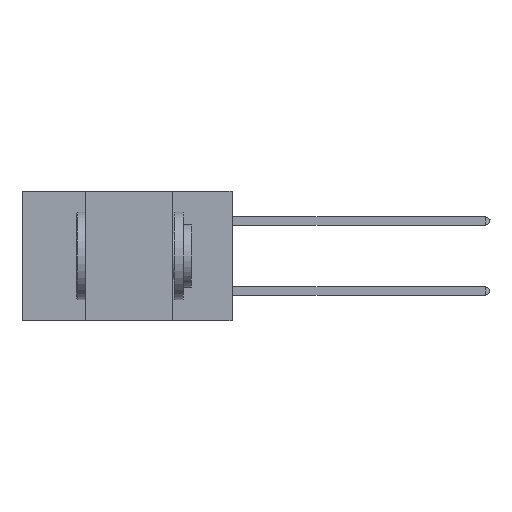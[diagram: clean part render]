
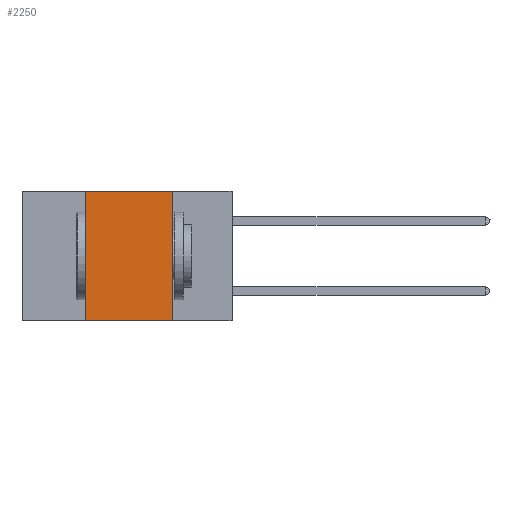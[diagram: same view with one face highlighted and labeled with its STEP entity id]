
A CAD part, left-side view. The second image highlights one B-rep face of the part: STEP entity #2250.
In plain terms, the highlighted planar face has unit normal (-1, 0, 0).
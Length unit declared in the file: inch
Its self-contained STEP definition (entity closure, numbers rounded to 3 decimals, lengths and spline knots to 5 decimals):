
#39 = CARTESIAN_POINT ( 'NONE',  ( 0., 0.17, -0.37 ) ) ;
#564 = ORIENTED_EDGE ( 'NONE', *, *, #9642, .F. ) ;
#655 = VECTOR ( 'NONE', #10500, 39.37008 ) ;
#731 = VERTEX_POINT ( 'NONE', #39 ) ;
#1164 = ORIENTED_EDGE ( 'NONE', *, *, #5326, .F. ) ;
#1680 = ORIENTED_EDGE ( 'NONE', *, *, #9008, .T. ) ;
#2250 = ADVANCED_FACE ( 'NONE', ( #8075 ), #3520, .F. ) ;
#2349 = EDGE_CURVE ( 'NONE', #7176, #6942, #9381, .T. ) ;
#2686 = DIRECTION ( 'NONE',  ( 0., 0., -1. ) ) ;
#2958 = VECTOR ( 'NONE', #10139, 39.37008 ) ;
#3029 = DIRECTION ( 'NONE',  ( 0., 0., 1. ) ) ;
#3080 = VECTOR ( 'NONE', #2686, 39.37008 ) ;
#3149 = EDGE_LOOP ( 'NONE', ( #564, #1164, #5261, #1680 ) ) ;
#3520 = PLANE ( 'NONE',  #9541 ) ;
#4089 = CARTESIAN_POINT ( 'NONE',  ( 0., 0.42, 0. ) ) ;
#4205 = CARTESIAN_POINT ( 'NONE',  ( 0., 0.42, 0. ) ) ;
#5202 = CARTESIAN_POINT ( 'NONE',  ( 0., 0.6, 0. ) ) ;
#5261 = ORIENTED_EDGE ( 'NONE', *, *, #2349, .F. ) ;
#5326 = EDGE_CURVE ( 'NONE', #6942, #9904, #7700, .T. ) ;
#5438 = LINE ( 'NONE', #7901, #3080 ) ;
#6510 = DIRECTION ( 'NONE',  ( 0., 0., -1. ) ) ;
#6512 = DIRECTION ( 'NONE',  ( 1., 0., 0. ) ) ;
#6942 = VERTEX_POINT ( 'NONE', #4205 ) ;
#7176 = VERTEX_POINT ( 'NONE', #9495 ) ;
#7332 = VECTOR ( 'NONE', #3029, 39.37008 ) ;
#7700 = LINE ( 'NONE', #9699, #655 ) ;
#7901 = CARTESIAN_POINT ( 'NONE',  ( 0., 0.17, 0. ) ) ;
#8075 = FACE_OUTER_BOUND ( 'NONE', #3149, .T. ) ;
#8216 = CARTESIAN_POINT ( 'NONE',  ( 0., 0.17, 0. ) ) ;
#9008 = EDGE_CURVE ( 'NONE', #7176, #731, #9663, .T. ) ;
#9333 = CARTESIAN_POINT ( 'NONE',  ( 0., 0.6, -0.37 ) ) ;
#9381 = LINE ( 'NONE', #4089, #7332 ) ;
#9495 = CARTESIAN_POINT ( 'NONE',  ( 0., 0.42, -0.37 ) ) ;
#9541 = AXIS2_PLACEMENT_3D ( 'NONE', #5202, #6512, #6510 ) ;
#9642 = EDGE_CURVE ( 'NONE', #9904, #731, #5438, .T. ) ;
#9663 = LINE ( 'NONE', #9333, #2958 ) ;
#9699 = CARTESIAN_POINT ( 'NONE',  ( 0., 0.6, 0. ) ) ;
#9904 = VERTEX_POINT ( 'NONE', #8216 ) ;
#10139 = DIRECTION ( 'NONE',  ( 0., -1., 0. ) ) ;
#10500 = DIRECTION ( 'NONE',  ( 0., -1., 0. ) ) ;
